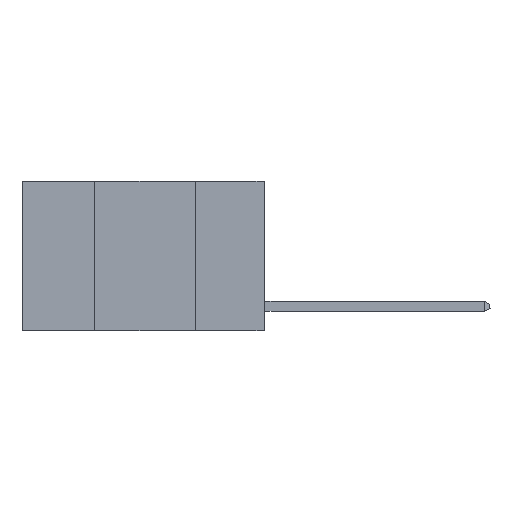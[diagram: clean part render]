
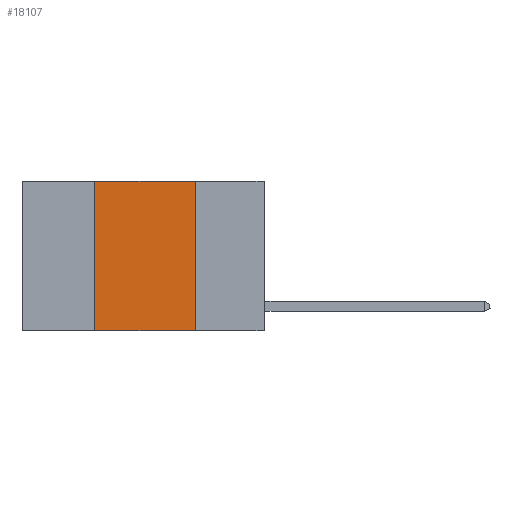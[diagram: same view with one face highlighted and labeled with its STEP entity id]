
A CAD part, left-side view. The second image highlights one B-rep face of the part: STEP entity #18107.
In plain terms, the highlighted planar face has unit normal (-1, 0, 0).
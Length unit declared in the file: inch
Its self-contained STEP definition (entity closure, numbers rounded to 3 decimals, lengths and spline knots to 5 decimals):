
#705 = VECTOR ( 'NONE', #4068, 39.37008 ) ;
#1445 = EDGE_LOOP ( 'NONE', ( #15043, #9178, #7856, #14509 ) ) ;
#1772 = EDGE_CURVE ( 'NONE', #14963, #3424, #13564, .T. ) ;
#3424 = VERTEX_POINT ( 'NONE', #7883 ) ;
#4068 = DIRECTION ( 'NONE',  ( 0., -1., 0. ) ) ;
#4702 = VERTEX_POINT ( 'NONE', #9574 ) ;
#4770 = AXIS2_PLACEMENT_3D ( 'NONE', #16645, #11832, #8607 ) ;
#4917 = DIRECTION ( 'NONE',  ( 0., 0., -1. ) ) ;
#5428 = PLANE ( 'NONE',  #4770 ) ;
#6987 = CARTESIAN_POINT ( 'NONE',  ( 0., 0.6, 0. ) ) ;
#7198 = CARTESIAN_POINT ( 'NONE',  ( 0., 0.42, -0.37 ) ) ;
#7497 = VECTOR ( 'NONE', #4917, 39.37008 ) ;
#7650 = LINE ( 'NONE', #6987, #11190 ) ;
#7856 = ORIENTED_EDGE ( 'NONE', *, *, #20529, .F. ) ;
#7883 = CARTESIAN_POINT ( 'NONE',  ( 0., 0.17, -0.37 ) ) ;
#8607 = DIRECTION ( 'NONE',  ( 0., 0., -1. ) ) ;
#9145 = LINE ( 'NONE', #13589, #705 ) ;
#9178 = ORIENTED_EDGE ( 'NONE', *, *, #16144, .F. ) ;
#9574 = CARTESIAN_POINT ( 'NONE',  ( 0., 0.42, 0. ) ) ;
#10004 = DIRECTION ( 'NONE',  ( 0., -1., 0. ) ) ;
#11190 = VECTOR ( 'NONE', #10004, 39.37008 ) ;
#11832 = DIRECTION ( 'NONE',  ( 1., 0., 0. ) ) ;
#13564 = LINE ( 'NONE', #14255, #7497 ) ;
#13589 = CARTESIAN_POINT ( 'NONE',  ( 0., 0.6, -0.37 ) ) ;
#13829 = VECTOR ( 'NONE', #20534, 39.37008 ) ;
#14114 = VERTEX_POINT ( 'NONE', #7198 ) ;
#14255 = CARTESIAN_POINT ( 'NONE',  ( 0., 0.17, 0. ) ) ;
#14509 = ORIENTED_EDGE ( 'NONE', *, *, #16693, .T. ) ;
#14847 = FACE_OUTER_BOUND ( 'NONE', #1445, .T. ) ;
#14963 = VERTEX_POINT ( 'NONE', #17483 ) ;
#15043 = ORIENTED_EDGE ( 'NONE', *, *, #1772, .F. ) ;
#16144 = EDGE_CURVE ( 'NONE', #4702, #14963, #7650, .T. ) ;
#16645 = CARTESIAN_POINT ( 'NONE',  ( 0., 0.6, 0. ) ) ;
#16693 = EDGE_CURVE ( 'NONE', #14114, #3424, #9145, .T. ) ;
#17483 = CARTESIAN_POINT ( 'NONE',  ( 0., 0.17, 0. ) ) ;
#18107 = ADVANCED_FACE ( 'NONE', ( #14847 ), #5428, .F. ) ;
#20489 = LINE ( 'NONE', #20604, #13829 ) ;
#20529 = EDGE_CURVE ( 'NONE', #14114, #4702, #20489, .T. ) ;
#20534 = DIRECTION ( 'NONE',  ( 0., 0., 1. ) ) ;
#20604 = CARTESIAN_POINT ( 'NONE',  ( 0., 0.42, 0. ) ) ;
